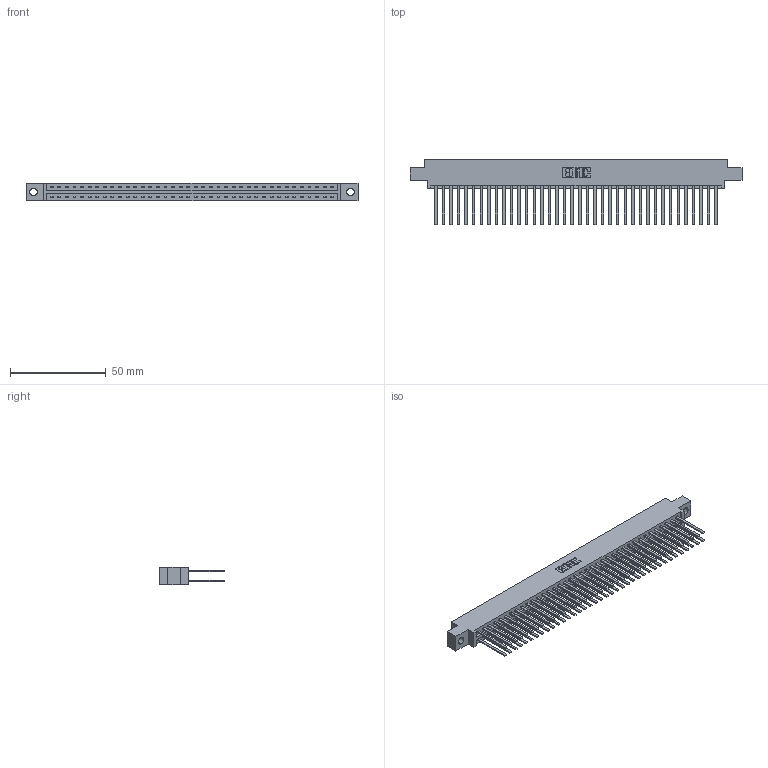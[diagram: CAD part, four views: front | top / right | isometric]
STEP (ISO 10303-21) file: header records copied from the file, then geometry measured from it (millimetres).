
FILE_DESCRIPTION (( 'STEP AP203' ), '1' );
FILE_NAME ('337-076-544-804.STEP', '2019-10-15T13:30:35', ( '' ), ( '' ), 'SwSTEP 2.0', 'SolidWorks 2016', '' );
FILE_SCHEMA (( 'CONFIG_CONTROL_DESIGN' ));
Length unit declared in the file: inch
Products named in the file (3): 345-292-001_345-293-144; 337 Part_0.170 Offset - 0.156 Dia-TH; 337-076-544-804
Assembly tree (77 placements, depth 2):
  337-076-544-804
    337 Part_0.170 Offset - 0.156 Dia-TH
    345-292-001_345-293-144  x76
Bounding box: 173.58 x 34.3 x 9.4 mm (x, y, z)
Volume: 19100.4 mm3; surface area: 24939.7 mm2
Topology: 77 solids, 77 shells, 3766 faces, 11191 edges, 7358 vertices
Faces by surface type: plane 2658, cylinder 1108
Entity records: 29931 total; most frequent: CARTESIAN_POINT 5046, ORIENTED_EDGE 4982, DIRECTION 4295, EDGE_CURVE 2491, LINE 2367, VECTOR 2367, VERTEX_POINT 1658, AXIS2_PLACEMENT_3D 964
